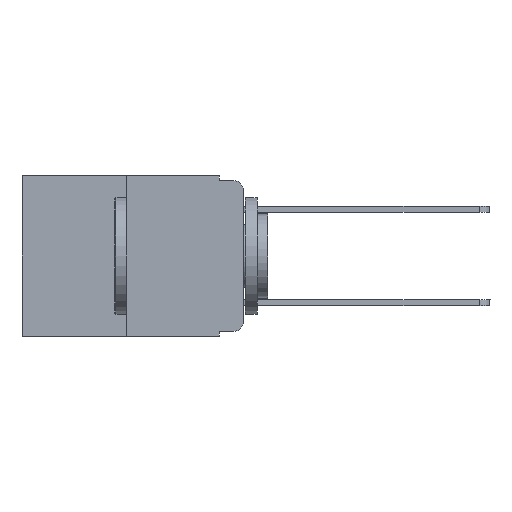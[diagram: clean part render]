
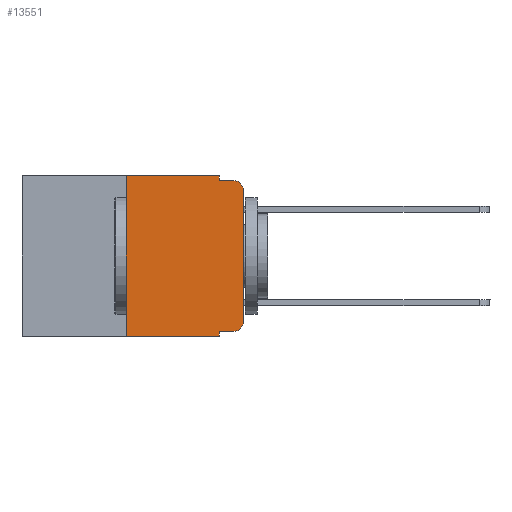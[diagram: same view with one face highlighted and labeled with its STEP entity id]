
A CAD part, left-side view. The second image highlights one B-rep face of the part: STEP entity #13551.
In plain terms, the highlighted planar face has unit normal (-1, 0, 0).
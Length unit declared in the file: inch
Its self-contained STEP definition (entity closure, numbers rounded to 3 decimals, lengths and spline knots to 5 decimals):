
#3 = CARTESIAN_POINT ( 'NONE',  ( 0., 0.25, 0. ) ) ;
#346 = EDGE_CURVE ( 'NONE', #1984, #11763, #9293, .T. ) ;
#387 = CARTESIAN_POINT ( 'NONE',  ( 0., 0., -0.313 ) ) ;
#456 = VERTEX_POINT ( 'NONE', #6086 ) ;
#511 = PLANE ( 'NONE',  #9834 ) ;
#658 = DIRECTION ( 'NONE',  ( 1., 0., 0. ) ) ;
#786 = VERTEX_POINT ( 'NONE', #11638 ) ;
#958 = ORIENTED_EDGE ( 'NONE', *, *, #7401, .T. ) ;
#1034 = VECTOR ( 'NONE', #8422, 39.37008 ) ;
#1045 = AXIS2_PLACEMENT_3D ( 'NONE', #13724, #5878, #1349 ) ;
#1255 = DIRECTION ( 'NONE',  ( 0., 0., 1. ) ) ;
#1297 = VERTEX_POINT ( 'NONE', #6184 ) ;
#1349 = DIRECTION ( 'NONE',  ( 0., 0., -1. ) ) ;
#1695 = VERTEX_POINT ( 'NONE', #10466 ) ;
#1984 = VERTEX_POINT ( 'NONE', #14002 ) ;
#2638 = LINE ( 'NONE', #7177, #14508 ) ;
#3236 = CARTESIAN_POINT ( 'NONE',  ( 0., 0.051, 0. ) ) ;
#3291 = ORIENTED_EDGE ( 'NONE', *, *, #9937, .F. ) ;
#4034 = EDGE_CURVE ( 'NONE', #14621, #786, #13276, .T. ) ;
#4288 = VERTEX_POINT ( 'NONE', #9635 ) ;
#4462 = CARTESIAN_POINT ( 'NONE',  ( 0., 0.25, -0.343 ) ) ;
#4601 = LINE ( 'NONE', #3, #11211 ) ;
#5113 = DIRECTION ( 'NONE',  ( 0., 0., -1. ) ) ;
#5296 = ORIENTED_EDGE ( 'NONE', *, *, #10850, .T. ) ;
#5436 = LINE ( 'NONE', #9961, #10293 ) ;
#5701 = VECTOR ( 'NONE', #13903, 39.37008 ) ;
#5787 = DIRECTION ( 'NONE',  ( 0., 0., 1. ) ) ;
#5814 = EDGE_CURVE ( 'NONE', #456, #786, #7637, .T. ) ;
#5878 = DIRECTION ( 'NONE',  ( -1., 0., 0. ) ) ;
#6082 = CARTESIAN_POINT ( 'NONE',  ( 0., 0.051, 0. ) ) ;
#6086 = CARTESIAN_POINT ( 'NONE',  ( 0., 0.051, -0.333 ) ) ;
#6184 = CARTESIAN_POINT ( 'NONE',  ( 0., 0.02, -0.01 ) ) ;
#6275 = VECTOR ( 'NONE', #5787, 39.37008 ) ;
#6377 = CARTESIAN_POINT ( 'NONE',  ( 0., 0.473, 0. ) ) ;
#6492 = ORIENTED_EDGE ( 'NONE', *, *, #11603, .F. ) ;
#6616 = VECTOR ( 'NONE', #12169, 39.37008 ) ;
#6685 = LINE ( 'NONE', #11203, #6275 ) ;
#6702 = AXIS2_PLACEMENT_3D ( 'NONE', #10532, #7348, #7135 ) ;
#7135 = DIRECTION ( 'NONE',  ( 0., 0., -1. ) ) ;
#7177 = CARTESIAN_POINT ( 'NONE',  ( 0., 0.051, 0. ) ) ;
#7348 = DIRECTION ( 'NONE',  ( -1., 0., 0. ) ) ;
#7401 = EDGE_CURVE ( 'NONE', #456, #1984, #11620, .T. ) ;
#7451 = CARTESIAN_POINT ( 'NONE',  ( 0., 0.051, -0.01 ) ) ;
#7475 = ORIENTED_EDGE ( 'NONE', *, *, #4034, .T. ) ;
#7637 = LINE ( 'NONE', #3236, #13271 ) ;
#7651 = CARTESIAN_POINT ( 'NONE',  ( 0., 0.473, -0.343 ) ) ;
#7818 = DIRECTION ( 'NONE',  ( 0., -1., 0. ) ) ;
#8000 = ORIENTED_EDGE ( 'NONE', *, *, #11323, .T. ) ;
#8159 = CIRCLE ( 'NONE', #1045, 0.02 ) ;
#8321 = ORIENTED_EDGE ( 'NONE', *, *, #5814, .F. ) ;
#8422 = DIRECTION ( 'NONE',  ( 0., -1., 0. ) ) ;
#8826 = VERTEX_POINT ( 'NONE', #12949 ) ;
#8891 = EDGE_CURVE ( 'NONE', #12276, #1695, #2638, .T. ) ;
#9293 = CIRCLE ( 'NONE', #6702, 0.02 ) ;
#9448 = LINE ( 'NONE', #7451, #1034 ) ;
#9635 = CARTESIAN_POINT ( 'NONE',  ( 0., 0.25, 0. ) ) ;
#9834 = AXIS2_PLACEMENT_3D ( 'NONE', #6377, #658, #5113 ) ;
#9937 = EDGE_CURVE ( 'NONE', #14621, #4288, #4601, .T. ) ;
#9961 = CARTESIAN_POINT ( 'NONE',  ( 0., 0.473, 0. ) ) ;
#10293 = VECTOR ( 'NONE', #7818, 39.37008 ) ;
#10466 = CARTESIAN_POINT ( 'NONE',  ( 0., 0.051, -0.01 ) ) ;
#10499 = EDGE_CURVE ( 'NONE', #1695, #1297, #9448, .T. ) ;
#10532 = CARTESIAN_POINT ( 'NONE',  ( 0., 0.02, -0.313 ) ) ;
#10641 = CARTESIAN_POINT ( 'NONE',  ( 0., 0.051, -0.333 ) ) ;
#10821 = FACE_OUTER_BOUND ( 'NONE', #11958, .T. ) ;
#10850 = EDGE_CURVE ( 'NONE', #8826, #1297, #8159, .T. ) ;
#11045 = DIRECTION ( 'NONE',  ( 0., 0., -1. ) ) ;
#11203 = CARTESIAN_POINT ( 'NONE',  ( 0., 0., 0. ) ) ;
#11211 = VECTOR ( 'NONE', #1255, 39.37008 ) ;
#11323 = EDGE_CURVE ( 'NONE', #11763, #8826, #6685, .T. ) ;
#11480 = ORIENTED_EDGE ( 'NONE', *, *, #346, .T. ) ;
#11603 = EDGE_CURVE ( 'NONE', #4288, #12276, #5436, .T. ) ;
#11620 = LINE ( 'NONE', #10641, #5701 ) ;
#11638 = CARTESIAN_POINT ( 'NONE',  ( 0., 0.051, -0.343 ) ) ;
#11696 = DIRECTION ( 'NONE',  ( 0., 0., -1. ) ) ;
#11763 = VERTEX_POINT ( 'NONE', #387 ) ;
#11777 = ORIENTED_EDGE ( 'NONE', *, *, #10499, .F. ) ;
#11958 = EDGE_LOOP ( 'NONE', ( #8000, #5296, #11777, #12121, #6492, #3291, #7475, #8321, #958, #11480 ) ) ;
#12121 = ORIENTED_EDGE ( 'NONE', *, *, #8891, .F. ) ;
#12169 = DIRECTION ( 'NONE',  ( 0., -1., 0. ) ) ;
#12276 = VERTEX_POINT ( 'NONE', #6082 ) ;
#12949 = CARTESIAN_POINT ( 'NONE',  ( 0., 0., -0.03 ) ) ;
#13271 = VECTOR ( 'NONE', #11045, 39.37008 ) ;
#13276 = LINE ( 'NONE', #7651, #6616 ) ;
#13551 = ADVANCED_FACE ( 'NONE', ( #10821 ), #511, .F. ) ;
#13724 = CARTESIAN_POINT ( 'NONE',  ( 0., 0.02, -0.03 ) ) ;
#13903 = DIRECTION ( 'NONE',  ( 0., -1., 0. ) ) ;
#14002 = CARTESIAN_POINT ( 'NONE',  ( 0., 0.02, -0.333 ) ) ;
#14508 = VECTOR ( 'NONE', #11696, 39.37008 ) ;
#14621 = VERTEX_POINT ( 'NONE', #4462 ) ;
